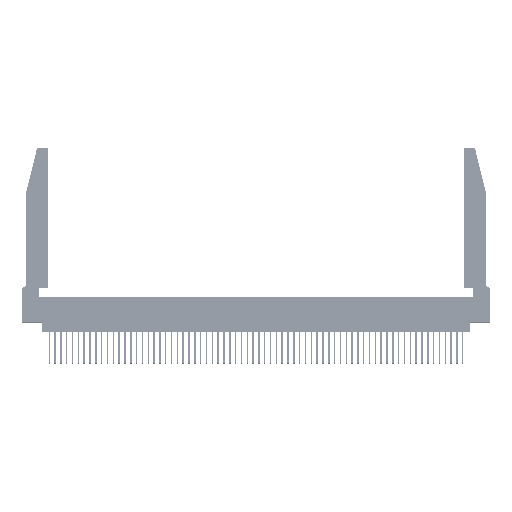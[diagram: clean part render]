
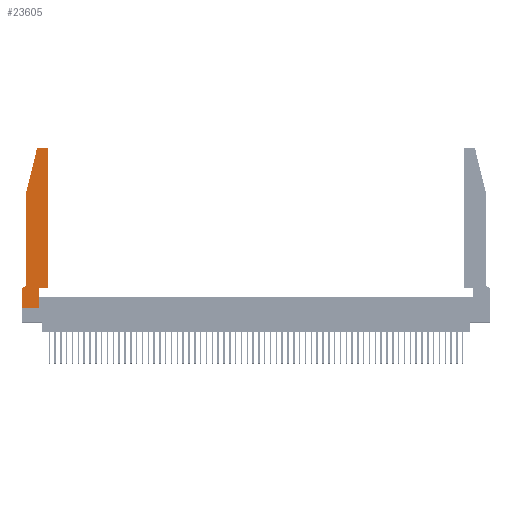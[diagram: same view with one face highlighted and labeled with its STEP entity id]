
A CAD part, top view. The second image highlights one B-rep face of the part: STEP entity #23605.
In plain terms, the highlighted planar face has unit normal (0, 0, 1).
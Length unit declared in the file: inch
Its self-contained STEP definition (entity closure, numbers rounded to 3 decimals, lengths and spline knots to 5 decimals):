
#2084 = ORIENTED_EDGE ( 'NONE', *, *, #34103, .T. ) ;
#3142 = CARTESIAN_POINT ( 'NONE',  ( 0.4205, 2.72, 0.37 ) ) ;
#3346 = EDGE_CURVE ( 'NONE', #50547, #41174, #14163, .T. ) ;
#4399 = LINE ( 'NONE', #48835, #35562 ) ;
#4701 = VERTEX_POINT ( 'NONE', #34395 ) ;
#5972 = VERTEX_POINT ( 'NONE', #57384 ) ;
#6605 = FACE_OUTER_BOUND ( 'NONE', #15976, .T. ) ;
#8072 = VERTEX_POINT ( 'NONE', #14228 ) ;
#8817 = DIRECTION ( 'NONE',  ( 1., 0., 0. ) ) ;
#10778 = AXIS2_PLACEMENT_3D ( 'NONE', #13014, #17450, #51860 ) ;
#11054 = CARTESIAN_POINT ( 'NONE',  ( 0.2865, 0.35, 0.37 ) ) ;
#11904 = DIRECTION ( 'NONE',  ( 1., 0., 0. ) ) ;
#12004 = CARTESIAN_POINT ( 'NONE',  ( 0.4505, 2.72, 0.37 ) ) ;
#12528 = VECTOR ( 'NONE', #54369, 39.37008 ) ;
#12847 = AXIS2_PLACEMENT_3D ( 'NONE', #25558, #56499, #48129 ) ;
#12918 = CARTESIAN_POINT ( 'NONE',  ( 0., 0., 0.37 ) ) ;
#13014 = CARTESIAN_POINT ( 'NONE',  ( 0., 0.35, 0.37 ) ) ;
#13145 = CARTESIAN_POINT ( 'NONE',  ( 0.4505, 0.35, 0.37 ) ) ;
#14163 = LINE ( 'NONE', #46297, #52872 ) ;
#14228 = CARTESIAN_POINT ( 'NONE',  ( 0.2865, 0.35, 0.37 ) ) ;
#14267 = ORIENTED_EDGE ( 'NONE', *, *, #3346, .T. ) ;
#15517 = EDGE_CURVE ( 'NONE', #4701, #22606, #52475, .T. ) ;
#15976 = EDGE_LOOP ( 'NONE', ( #26463, #57196, #51796, #52980, #19868, #18546, #34211, #14267, #56283, #28960, #2084, #36224 ) ) ;
#17450 = DIRECTION ( 'NONE',  ( 0., 0., 1. ) ) ;
#18546 = ORIENTED_EDGE ( 'NONE', *, *, #46505, .T. ) ;
#18993 = CARTESIAN_POINT ( 'NONE',  ( 0.2605, 2.75, 0.37 ) ) ;
#19868 = ORIENTED_EDGE ( 'NONE', *, *, #38948, .T. ) ;
#21217 = VECTOR ( 'NONE', #29047, 39.37008 ) ;
#21250 = DIRECTION ( 'NONE',  ( -0.239, -0.971, 0. ) ) ;
#21930 = CIRCLE ( 'NONE', #23853, 0.03 ) ;
#22033 = LINE ( 'NONE', #52784, #46907 ) ;
#22606 = VERTEX_POINT ( 'NONE', #45954 ) ;
#23605 = ADVANCED_FACE ( 'NONE', ( #6605 ), #39419, .T. ) ;
#23853 = AXIS2_PLACEMENT_3D ( 'NONE', #3142, #42988, #11904 ) ;
#25558 = CARTESIAN_POINT ( 'NONE',  ( 0.0055, 0.42, 0.37 ) ) ;
#26463 = ORIENTED_EDGE ( 'NONE', *, *, #33638, .T. ) ;
#27702 = EDGE_CURVE ( 'NONE', #42206, #4701, #42325, .T. ) ;
#28247 = CARTESIAN_POINT ( 'NONE',  ( 0.2865, 0., 0.37 ) ) ;
#28349 = DIRECTION ( 'NONE',  ( 1., 0., 0. ) ) ;
#28960 = ORIENTED_EDGE ( 'NONE', *, *, #56123, .T. ) ;
#29047 = DIRECTION ( 'NONE',  ( 0., 1., 0. ) ) ;
#29074 = VERTEX_POINT ( 'NONE', #36438 ) ;
#30132 = CARTESIAN_POINT ( 'NONE',  ( 0.0755, 2., 0.37 ) ) ;
#30330 = CARTESIAN_POINT ( 'NONE',  ( 0., 0.35, 0.37 ) ) ;
#31045 = EDGE_CURVE ( 'NONE', #45033, #50547, #37780, .T. ) ;
#33638 = EDGE_CURVE ( 'NONE', #38682, #42206, #36031, .T. ) ;
#33686 = VECTOR ( 'NONE', #38882, 39.37008 ) ;
#33694 = VECTOR ( 'NONE', #40919, 39.37008 ) ;
#34103 = EDGE_CURVE ( 'NONE', #5972, #54499, #51216, .T. ) ;
#34211 = ORIENTED_EDGE ( 'NONE', *, *, #31045, .T. ) ;
#34395 = CARTESIAN_POINT ( 'NONE',  ( 0.25487, 2.72718, 0.37 ) ) ;
#34525 = VECTOR ( 'NONE', #21250, 39.37008 ) ;
#34788 = DIRECTION ( 'NONE',  ( 0., 1., 0. ) ) ;
#35562 = VECTOR ( 'NONE', #8817, 39.37008 ) ;
#36031 = LINE ( 'NONE', #18993, #12528 ) ;
#36224 = ORIENTED_EDGE ( 'NONE', *, *, #47601, .T. ) ;
#36438 = CARTESIAN_POINT ( 'NONE',  ( 0.0055, 0.35, 0.37 ) ) ;
#36458 = EDGE_CURVE ( 'NONE', #22606, #39542, #46074, .T. ) ;
#36502 = AXIS2_PLACEMENT_3D ( 'NONE', #53639, #53447, #44330 ) ;
#37780 = LINE ( 'NONE', #54511, #33694 ) ;
#38045 = VECTOR ( 'NONE', #34788, 39.37008 ) ;
#38175 = CIRCLE ( 'NONE', #12847, 0.07 ) ;
#38682 = VERTEX_POINT ( 'NONE', #41551 ) ;
#38882 = DIRECTION ( 'NONE',  ( 0., -1., 0. ) ) ;
#38948 = EDGE_CURVE ( 'NONE', #39542, #29074, #38175, .T. ) ;
#39419 = PLANE ( 'NONE',  #10778 ) ;
#39542 = VERTEX_POINT ( 'NONE', #47912 ) ;
#40919 = DIRECTION ( 'NONE',  ( 0., -1., 0. ) ) ;
#41174 = VERTEX_POINT ( 'NONE', #28247 ) ;
#41551 = CARTESIAN_POINT ( 'NONE',  ( 0.4205, 2.75, 0.37 ) ) ;
#42206 = VERTEX_POINT ( 'NONE', #52311 ) ;
#42325 = CIRCLE ( 'NONE', #36502, 0.03 ) ;
#42988 = DIRECTION ( 'NONE',  ( 0., 0., 1. ) ) ;
#43520 = CARTESIAN_POINT ( 'NONE',  ( 0.0755, 2., 0.37 ) ) ;
#44330 = DIRECTION ( 'NONE',  ( 1., 0., 0. ) ) ;
#45033 = VERTEX_POINT ( 'NONE', #30330 ) ;
#45954 = CARTESIAN_POINT ( 'NONE',  ( 0.0755, 2., 0.37 ) ) ;
#46074 = LINE ( 'NONE', #43520, #33686 ) ;
#46094 = LINE ( 'NONE', #11054, #21217 ) ;
#46297 = CARTESIAN_POINT ( 'NONE',  ( 0., 0., 0.37 ) ) ;
#46505 = EDGE_CURVE ( 'NONE', #29074, #45033, #22033, .T. ) ;
#46907 = VECTOR ( 'NONE', #47950, 39.37008 ) ;
#47601 = EDGE_CURVE ( 'NONE', #54499, #38682, #21930, .T. ) ;
#47912 = CARTESIAN_POINT ( 'NONE',  ( 0.0755, 0.42, 0.37 ) ) ;
#47950 = DIRECTION ( 'NONE',  ( -1., 0., 0. ) ) ;
#48129 = DIRECTION ( 'NONE',  ( -1., 0., 0. ) ) ;
#48835 = CARTESIAN_POINT ( 'NONE',  ( 0.4505, 0.35, 0.37 ) ) ;
#50547 = VERTEX_POINT ( 'NONE', #12918 ) ;
#51216 = LINE ( 'NONE', #13145, #38045 ) ;
#51796 = ORIENTED_EDGE ( 'NONE', *, *, #15517, .T. ) ;
#51860 = DIRECTION ( 'NONE',  ( 1., 0., 0. ) ) ;
#52311 = CARTESIAN_POINT ( 'NONE',  ( 0.284, 2.75, 0.37 ) ) ;
#52475 = LINE ( 'NONE', #30132, #34525 ) ;
#52784 = CARTESIAN_POINT ( 'NONE',  ( 0.0755, 0.35, 0.37 ) ) ;
#52872 = VECTOR ( 'NONE', #28349, 39.37008 ) ;
#52980 = ORIENTED_EDGE ( 'NONE', *, *, #36458, .T. ) ;
#53447 = DIRECTION ( 'NONE',  ( 0., 0., 1. ) ) ;
#53639 = CARTESIAN_POINT ( 'NONE',  ( 0.284, 2.72, 0.37 ) ) ;
#54369 = DIRECTION ( 'NONE',  ( -1., 0., 0. ) ) ;
#54499 = VERTEX_POINT ( 'NONE', #12004 ) ;
#54511 = CARTESIAN_POINT ( 'NONE',  ( 0., 0., 0.37 ) ) ;
#55085 = EDGE_CURVE ( 'NONE', #41174, #8072, #46094, .T. ) ;
#56123 = EDGE_CURVE ( 'NONE', #8072, #5972, #4399, .T. ) ;
#56283 = ORIENTED_EDGE ( 'NONE', *, *, #55085, .T. ) ;
#56499 = DIRECTION ( 'NONE',  ( 0., 0., -1. ) ) ;
#57196 = ORIENTED_EDGE ( 'NONE', *, *, #27702, .T. ) ;
#57384 = CARTESIAN_POINT ( 'NONE',  ( 0.4505, 0.35, 0.37 ) ) ;
